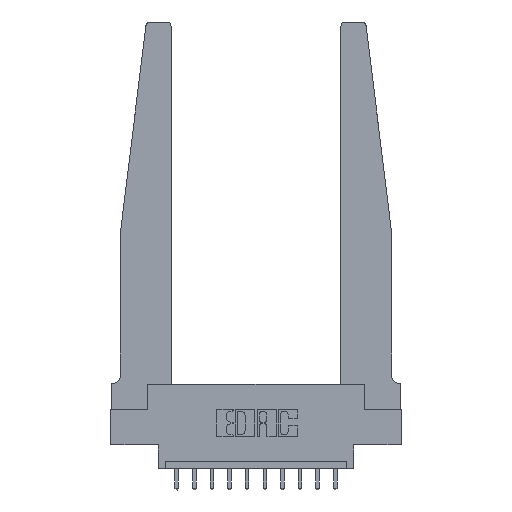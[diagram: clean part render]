
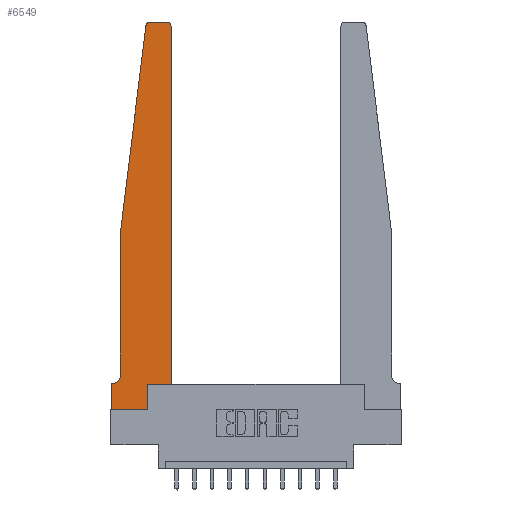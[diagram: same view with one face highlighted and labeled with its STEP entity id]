
A CAD part, top view. The second image highlights one B-rep face of the part: STEP entity #6549.
In plain terms, the highlighted planar face has unit normal (0, 0, 1).
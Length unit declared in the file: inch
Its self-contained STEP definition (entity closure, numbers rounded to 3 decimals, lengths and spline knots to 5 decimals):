
#369 = CARTESIAN_POINT ( 'NONE',  ( 0., 0., 0.37 ) ) ;
#463 = VERTEX_POINT ( 'NONE', #11767 ) ;
#770 = DIRECTION ( 'NONE',  ( 1., 0., 0. ) ) ;
#1176 = CARTESIAN_POINT ( 'NONE',  ( 0.065, 1.25, 0.37 ) ) ;
#1559 = VECTOR ( 'NONE', #2033, 39.37008 ) ;
#1600 = CARTESIAN_POINT ( 'NONE',  ( 0.24675, 2.72367, 0.37 ) ) ;
#1938 = ORIENTED_EDGE ( 'NONE', *, *, #15245, .T. ) ;
#1954 = ORIENTED_EDGE ( 'NONE', *, *, #6071, .T. ) ;
#1995 = LINE ( 'NONE', #3629, #10204 ) ;
#1997 = VERTEX_POINT ( 'NONE', #6674 ) ;
#2002 = VECTOR ( 'NONE', #7842, 39.37008 ) ;
#2033 = DIRECTION ( 'NONE',  ( -1., 0., 0. ) ) ;
#2374 = ORIENTED_EDGE ( 'NONE', *, *, #6392, .T. ) ;
#2394 = DIRECTION ( 'NONE',  ( 1., 0., 0. ) ) ;
#2670 = DIRECTION ( 'NONE',  ( 1., 0., 0. ) ) ;
#2692 = EDGE_CURVE ( 'NONE', #15084, #6812, #3579, .T. ) ;
#2941 = CARTESIAN_POINT ( 'NONE',  ( 0., 0., 0.37 ) ) ;
#3079 = CARTESIAN_POINT ( 'NONE',  ( 0.425, 0.18, 0.37 ) ) ;
#3340 = DIRECTION ( 'NONE',  ( -1., 0., 0. ) ) ;
#3369 = VERTEX_POINT ( 'NONE', #10082 ) ;
#3494 = AXIS2_PLACEMENT_3D ( 'NONE', #9435, #8405, #2394 ) ;
#3579 = LINE ( 'NONE', #369, #11818 ) ;
#3629 = CARTESIAN_POINT ( 'NONE',  ( 0.2605, 0.18, 0.37 ) ) ;
#3671 = LINE ( 'NONE', #2941, #2002 ) ;
#3748 = EDGE_CURVE ( 'NONE', #13897, #11882, #1995, .T. ) ;
#3754 = AXIS2_PLACEMENT_3D ( 'NONE', #10872, #12126, #2670 ) ;
#4348 = CIRCLE ( 'NONE', #3754, 0.03 ) ;
#4363 = ORIENTED_EDGE ( 'NONE', *, *, #3748, .T. ) ;
#4703 = CARTESIAN_POINT ( 'NONE',  ( 0.015, 0.2375, 0.37 ) ) ;
#5782 = LINE ( 'NONE', #10678, #11189 ) ;
#5937 = PLANE ( 'NONE',  #3494 ) ;
#5940 = LINE ( 'NONE', #14446, #7055 ) ;
#5946 = CARTESIAN_POINT ( 'NONE',  ( 0.425, 0.18, 0.37 ) ) ;
#6071 = EDGE_CURVE ( 'NONE', #1997, #11393, #7903, .T. ) ;
#6292 = CARTESIAN_POINT ( 'NONE',  ( 0., 0., 0.37 ) ) ;
#6392 = EDGE_CURVE ( 'NONE', #3369, #463, #14628, .T. ) ;
#6549 = ADVANCED_FACE ( 'NONE', ( #11999 ), #5937, .T. ) ;
#6646 = CARTESIAN_POINT ( 'NONE',  ( 0.015, 0.1875, 0.37 ) ) ;
#6674 = CARTESIAN_POINT ( 'NONE',  ( 0.065, 0.2375, 0.37 ) ) ;
#6812 = VERTEX_POINT ( 'NONE', #6292 ) ;
#6876 = LINE ( 'NONE', #15083, #15109 ) ;
#7039 = DIRECTION ( 'NONE',  ( 0., 0., -1. ) ) ;
#7055 = VECTOR ( 'NONE', #10738, 39.37008 ) ;
#7271 = ORIENTED_EDGE ( 'NONE', *, *, #7801, .T. ) ;
#7314 = VERTEX_POINT ( 'NONE', #1600 ) ;
#7801 = EDGE_CURVE ( 'NONE', #7314, #14750, #5782, .T. ) ;
#7842 = DIRECTION ( 'NONE',  ( 1., 0., 0. ) ) ;
#7903 = CIRCLE ( 'NONE', #15079, 0.05 ) ;
#7972 = CARTESIAN_POINT ( 'NONE',  ( 0.25, 2.75, 0.37 ) ) ;
#7981 = CIRCLE ( 'NONE', #8335, 0.03 ) ;
#8335 = AXIS2_PLACEMENT_3D ( 'NONE', #12627, #9093, #770 ) ;
#8405 = DIRECTION ( 'NONE',  ( 0., 0., 1. ) ) ;
#8431 = ORIENTED_EDGE ( 'NONE', *, *, #11641, .T. ) ;
#8551 = DIRECTION ( 'NONE',  ( 0., -1., 0. ) ) ;
#8556 = VERTEX_POINT ( 'NONE', #14680 ) ;
#8869 = EDGE_CURVE ( 'NONE', #14750, #1997, #12488, .T. ) ;
#9093 = DIRECTION ( 'NONE',  ( 0., 0., 1. ) ) ;
#9435 = CARTESIAN_POINT ( 'NONE',  ( 0., 0.1875, 0.37 ) ) ;
#9438 = DIRECTION ( 'NONE',  ( 0., -1., 0. ) ) ;
#9509 = VECTOR ( 'NONE', #12604, 39.37008 ) ;
#9781 = ORIENTED_EDGE ( 'NONE', *, *, #11388, .T. ) ;
#9914 = EDGE_CURVE ( 'NONE', #11393, #15084, #6876, .T. ) ;
#10070 = ORIENTED_EDGE ( 'NONE', *, *, #8869, .T. ) ;
#10076 = ORIENTED_EDGE ( 'NONE', *, *, #12343, .T. ) ;
#10082 = CARTESIAN_POINT ( 'NONE',  ( 0.395, 2.75, 0.37 ) ) ;
#10204 = VECTOR ( 'NONE', #10577, 39.37008 ) ;
#10577 = DIRECTION ( 'NONE',  ( 0., 1., 0. ) ) ;
#10678 = CARTESIAN_POINT ( 'NONE',  ( 0.065, 1.25, 0.37 ) ) ;
#10729 = DIRECTION ( 'NONE',  ( -0.122, -0.992, 0. ) ) ;
#10738 = DIRECTION ( 'NONE',  ( 0., 1., 0. ) ) ;
#10872 = CARTESIAN_POINT ( 'NONE',  ( 0.27653, 2.72, 0.37 ) ) ;
#10961 = VERTEX_POINT ( 'NONE', #5946 ) ;
#11189 = VECTOR ( 'NONE', #10729, 39.37008 ) ;
#11388 = EDGE_CURVE ( 'NONE', #11882, #10961, #13062, .T. ) ;
#11393 = VERTEX_POINT ( 'NONE', #6646 ) ;
#11515 = CARTESIAN_POINT ( 'NONE',  ( 0.2605, 0.18, 0.37 ) ) ;
#11641 = EDGE_CURVE ( 'NONE', #10961, #8556, #5940, .T. ) ;
#11767 = CARTESIAN_POINT ( 'NONE',  ( 0.27653, 2.75, 0.37 ) ) ;
#11818 = VECTOR ( 'NONE', #8551, 39.37008 ) ;
#11882 = VERTEX_POINT ( 'NONE', #11515 ) ;
#11930 = CARTESIAN_POINT ( 'NONE',  ( 0., 0.1875, 0.37 ) ) ;
#11989 = ORIENTED_EDGE ( 'NONE', *, *, #2692, .T. ) ;
#11999 = FACE_OUTER_BOUND ( 'NONE', #13631, .T. ) ;
#12126 = DIRECTION ( 'NONE',  ( 0., 0., 1. ) ) ;
#12200 = CARTESIAN_POINT ( 'NONE',  ( 0.065, 1.25, 0.37 ) ) ;
#12343 = EDGE_CURVE ( 'NONE', #8556, #3369, #7981, .T. ) ;
#12455 = EDGE_CURVE ( 'NONE', #6812, #13897, #3671, .T. ) ;
#12488 = LINE ( 'NONE', #1176, #13047 ) ;
#12604 = DIRECTION ( 'NONE',  ( 1., 0., 0. ) ) ;
#12627 = CARTESIAN_POINT ( 'NONE',  ( 0.395, 2.72, 0.37 ) ) ;
#12788 = CARTESIAN_POINT ( 'NONE',  ( 0.2605, 0., 0.37 ) ) ;
#13047 = VECTOR ( 'NONE', #9438, 39.37008 ) ;
#13062 = LINE ( 'NONE', #3079, #9509 ) ;
#13631 = EDGE_LOOP ( 'NONE', ( #2374, #1938, #7271, #10070, #1954, #13832, #11989, #13989, #4363, #9781, #8431, #10076 ) ) ;
#13832 = ORIENTED_EDGE ( 'NONE', *, *, #9914, .T. ) ;
#13897 = VERTEX_POINT ( 'NONE', #12788 ) ;
#13989 = ORIENTED_EDGE ( 'NONE', *, *, #12455, .T. ) ;
#14446 = CARTESIAN_POINT ( 'NONE',  ( 0.425, 0.18, 0.37 ) ) ;
#14628 = LINE ( 'NONE', #7972, #1559 ) ;
#14680 = CARTESIAN_POINT ( 'NONE',  ( 0.425, 2.72, 0.37 ) ) ;
#14750 = VERTEX_POINT ( 'NONE', #12200 ) ;
#15079 = AXIS2_PLACEMENT_3D ( 'NONE', #4703, #7039, #15302 ) ;
#15083 = CARTESIAN_POINT ( 'NONE',  ( 0.065, 0.1875, 0.37 ) ) ;
#15084 = VERTEX_POINT ( 'NONE', #11930 ) ;
#15109 = VECTOR ( 'NONE', #3340, 39.37008 ) ;
#15245 = EDGE_CURVE ( 'NONE', #463, #7314, #4348, .T. ) ;
#15302 = DIRECTION ( 'NONE',  ( -1., 0., 0. ) ) ;
